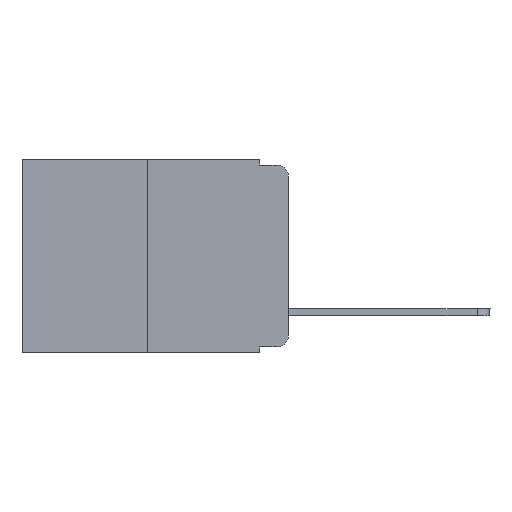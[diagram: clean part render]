
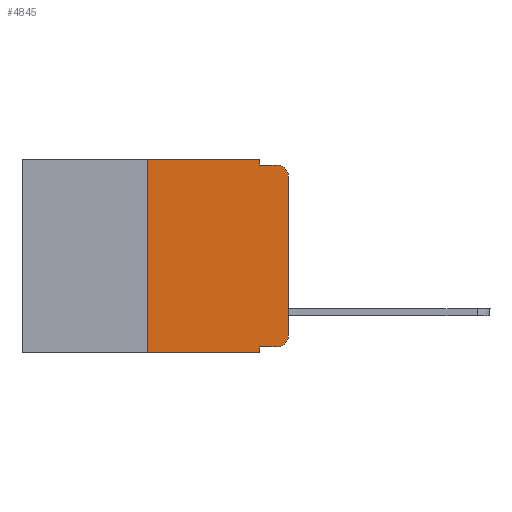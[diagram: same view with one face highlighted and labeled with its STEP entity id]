
A CAD part, left-side view. The second image highlights one B-rep face of the part: STEP entity #4845.
In plain terms, the highlighted planar face has unit normal (-1, 0, 0).
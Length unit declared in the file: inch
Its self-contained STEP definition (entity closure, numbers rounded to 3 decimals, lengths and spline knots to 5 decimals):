
#310 = VERTEX_POINT ( 'NONE', #13559 ) ;
#586 = LINE ( 'NONE', #11815, #3342 ) ;
#688 = VECTOR ( 'NONE', #16372, 39.37008 ) ;
#1189 = VERTEX_POINT ( 'NONE', #4620 ) ;
#1500 = CARTESIAN_POINT ( 'NONE',  ( 0., 0.25, 0. ) ) ;
#1752 = CIRCLE ( 'NONE', #2555, 0.02 ) ;
#2204 = LINE ( 'NONE', #13880, #9749 ) ;
#2508 = VECTOR ( 'NONE', #9595, 39.37008 ) ;
#2555 = AXIS2_PLACEMENT_3D ( 'NONE', #5318, #8987, #5468 ) ;
#2864 = CARTESIAN_POINT ( 'NONE',  ( 0., 0.02, -0.01 ) ) ;
#2908 = CARTESIAN_POINT ( 'NONE',  ( 0., 0.25, -0.343 ) ) ;
#2951 = CARTESIAN_POINT ( 'NONE',  ( 0., 0.051, -0.01 ) ) ;
#3342 = VECTOR ( 'NONE', #5446, 39.37008 ) ;
#3438 = CARTESIAN_POINT ( 'NONE',  ( 0., 0.051, -0.333 ) ) ;
#3521 = EDGE_CURVE ( 'NONE', #10418, #5227, #15498, .T. ) ;
#3595 = CARTESIAN_POINT ( 'NONE',  ( 0., 0.051, -0.343 ) ) ;
#3747 = EDGE_CURVE ( 'NONE', #310, #8793, #4612, .T. ) ;
#3857 = VERTEX_POINT ( 'NONE', #3595 ) ;
#3975 = VERTEX_POINT ( 'NONE', #1500 ) ;
#3980 = FACE_OUTER_BOUND ( 'NONE', #5825, .T. ) ;
#4053 = CARTESIAN_POINT ( 'NONE',  ( 0., 0.473, 0. ) ) ;
#4064 = LINE ( 'NONE', #5408, #8693 ) ;
#4612 = LINE ( 'NONE', #3438, #12323 ) ;
#4620 = CARTESIAN_POINT ( 'NONE',  ( 0., 0.051, -0.01 ) ) ;
#4632 = CARTESIAN_POINT ( 'NONE',  ( 0., 0., -0.03 ) ) ;
#4752 = ORIENTED_EDGE ( 'NONE', *, *, #14424, .T. ) ;
#4845 = ADVANCED_FACE ( 'NONE', ( #3980 ), #5152, .F. ) ;
#4964 = CARTESIAN_POINT ( 'NONE',  ( 0., 0.051, 0. ) ) ;
#4995 = EDGE_CURVE ( 'NONE', #1189, #13561, #15982, .T. ) ;
#5052 = LINE ( 'NONE', #7416, #688 ) ;
#5152 = PLANE ( 'NONE',  #15086 ) ;
#5183 = EDGE_CURVE ( 'NONE', #8793, #10418, #9225, .T. ) ;
#5227 = VERTEX_POINT ( 'NONE', #4632 ) ;
#5318 = CARTESIAN_POINT ( 'NONE',  ( 0., 0.02, -0.03 ) ) ;
#5408 = CARTESIAN_POINT ( 'NONE',  ( 0., 0.473, -0.343 ) ) ;
#5446 = DIRECTION ( 'NONE',  ( 0., 0., -1. ) ) ;
#5468 = DIRECTION ( 'NONE',  ( 0., 0., -1. ) ) ;
#5825 = EDGE_LOOP ( 'NONE', ( #11757, #13392, #15328, #12940, #9440, #6709, #4752, #8380, #7791, #10531 ) ) ;
#5906 = DIRECTION ( 'NONE',  ( -1., 0., 0. ) ) ;
#6050 = VECTOR ( 'NONE', #10671, 39.37008 ) ;
#6153 = DIRECTION ( 'NONE',  ( 0., 0., -1. ) ) ;
#6709 = ORIENTED_EDGE ( 'NONE', *, *, #16306, .F. ) ;
#7221 = CARTESIAN_POINT ( 'NONE',  ( 0., 0.02, -0.333 ) ) ;
#7416 = CARTESIAN_POINT ( 'NONE',  ( 0., 0.051, 0. ) ) ;
#7791 = ORIENTED_EDGE ( 'NONE', *, *, #3747, .T. ) ;
#8235 = EDGE_CURVE ( 'NONE', #310, #3857, #586, .T. ) ;
#8380 = ORIENTED_EDGE ( 'NONE', *, *, #8235, .F. ) ;
#8402 = CARTESIAN_POINT ( 'NONE',  ( 0., 0.25, 0. ) ) ;
#8693 = VECTOR ( 'NONE', #10518, 39.37008 ) ;
#8793 = VERTEX_POINT ( 'NONE', #7221 ) ;
#8987 = DIRECTION ( 'NONE',  ( -1., 0., 0. ) ) ;
#9225 = CIRCLE ( 'NONE', #13804, 0.02 ) ;
#9440 = ORIENTED_EDGE ( 'NONE', *, *, #13498, .F. ) ;
#9523 = CARTESIAN_POINT ( 'NONE',  ( 0., 0., -0.313 ) ) ;
#9595 = DIRECTION ( 'NONE',  ( 0., -1., 0. ) ) ;
#9749 = VECTOR ( 'NONE', #11344, 39.37008 ) ;
#9902 = DIRECTION ( 'NONE',  ( 0., -1., 0. ) ) ;
#10418 = VERTEX_POINT ( 'NONE', #9523 ) ;
#10518 = DIRECTION ( 'NONE',  ( 0., -1., 0. ) ) ;
#10531 = ORIENTED_EDGE ( 'NONE', *, *, #5183, .T. ) ;
#10671 = DIRECTION ( 'NONE',  ( 0., 0., 1. ) ) ;
#11337 = CARTESIAN_POINT ( 'NONE',  ( 0., 0.02, -0.313 ) ) ;
#11344 = DIRECTION ( 'NONE',  ( 0., -1., 0. ) ) ;
#11686 = DIRECTION ( 'NONE',  ( 0., 0., -1. ) ) ;
#11757 = ORIENTED_EDGE ( 'NONE', *, *, #3521, .T. ) ;
#11815 = CARTESIAN_POINT ( 'NONE',  ( 0., 0.051, 0. ) ) ;
#12323 = VECTOR ( 'NONE', #9902, 39.37008 ) ;
#12940 = ORIENTED_EDGE ( 'NONE', *, *, #15129, .F. ) ;
#13392 = ORIENTED_EDGE ( 'NONE', *, *, #16185, .T. ) ;
#13498 = EDGE_CURVE ( 'NONE', #3975, #15161, #2204, .T. ) ;
#13559 = CARTESIAN_POINT ( 'NONE',  ( 0., 0.051, -0.333 ) ) ;
#13561 = VERTEX_POINT ( 'NONE', #2864 ) ;
#13804 = AXIS2_PLACEMENT_3D ( 'NONE', #11337, #5906, #6153 ) ;
#13880 = CARTESIAN_POINT ( 'NONE',  ( 0., 0.473, 0. ) ) ;
#13911 = VERTEX_POINT ( 'NONE', #2908 ) ;
#14077 = DIRECTION ( 'NONE',  ( 0., 0., 1. ) ) ;
#14424 = EDGE_CURVE ( 'NONE', #13911, #3857, #4064, .T. ) ;
#14998 = VECTOR ( 'NONE', #14077, 39.37008 ) ;
#15086 = AXIS2_PLACEMENT_3D ( 'NONE', #4053, #15486, #11686 ) ;
#15129 = EDGE_CURVE ( 'NONE', #15161, #1189, #5052, .T. ) ;
#15161 = VERTEX_POINT ( 'NONE', #4964 ) ;
#15328 = ORIENTED_EDGE ( 'NONE', *, *, #4995, .F. ) ;
#15486 = DIRECTION ( 'NONE',  ( 1., 0., 0. ) ) ;
#15498 = LINE ( 'NONE', #16504, #14998 ) ;
#15982 = LINE ( 'NONE', #2951, #2508 ) ;
#16132 = LINE ( 'NONE', #8402, #6050 ) ;
#16185 = EDGE_CURVE ( 'NONE', #5227, #13561, #1752, .T. ) ;
#16306 = EDGE_CURVE ( 'NONE', #13911, #3975, #16132, .T. ) ;
#16372 = DIRECTION ( 'NONE',  ( 0., 0., -1. ) ) ;
#16504 = CARTESIAN_POINT ( 'NONE',  ( 0., 0., 0. ) ) ;
